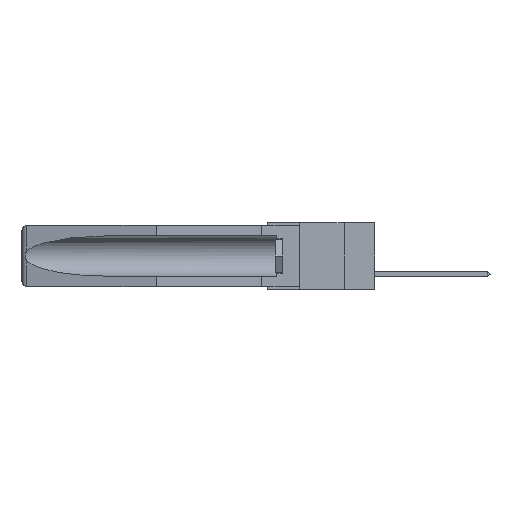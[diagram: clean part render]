
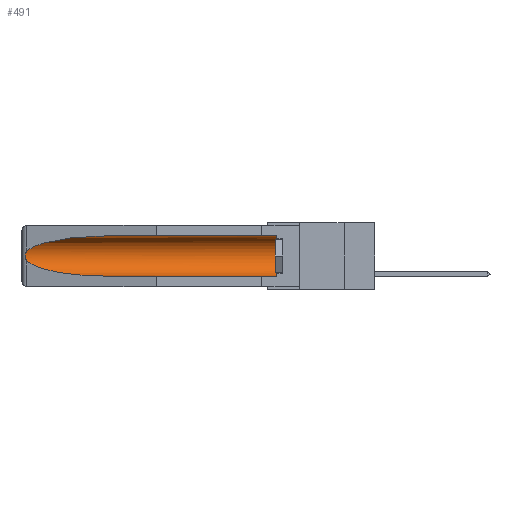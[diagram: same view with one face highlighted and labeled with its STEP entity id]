
A CAD part, left-side view. The second image highlights one B-rep face of the part: STEP entity #491.
In plain terms, the highlighted cylindrical face has radius 2.857 mm (diameter 5.715 mm), a partial arc.
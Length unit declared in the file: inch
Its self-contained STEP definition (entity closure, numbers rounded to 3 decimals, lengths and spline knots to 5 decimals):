
#352 = VERTEX_POINT ( 'NONE', #27739 ) ;
#491 = ADVANCED_FACE ( 'NONE', ( #23785 ), #9913, .F. ) ;
#625 =( BOUNDED_CURVE ( )  B_SPLINE_CURVE ( 3, ( #20214, #18277, #15750, #11184 ),
 .UNSPECIFIED., .F., .F. ) 
 B_SPLINE_CURVE_WITH_KNOTS ( ( 4, 4 ),
 ( 0.1948, 1.5708 ),
 .UNSPECIFIED. ) 
 CURVE ( )  GEOMETRIC_REPRESENTATION_ITEM ( )  RATIONAL_B_SPLINE_CURVE ( ( 1., 0.848, 0.848, 1. ) ) 
 REPRESENTATION_ITEM ( '' )  );
#1029 = DIRECTION ( 'NONE',  ( 0., -1., 0. ) ) ;
#1042 = CARTESIAN_POINT ( 'NONE',  ( 0.26537, 1.52718, -0.14972 ) ) ;
#1168 = CARTESIAN_POINT ( 'NONE',  ( 0.155, 0.126, -0.284 ) ) ;
#1497 = ORIENTED_EDGE ( 'NONE', *, *, #26198, .T. ) ;
#1573 = VECTOR ( 'NONE', #19853, 39.37008 ) ;
#1651 = LINE ( 'NONE', #2618, #8540 ) ;
#1716 = ORIENTED_EDGE ( 'NONE', *, *, #5373, .T. ) ;
#2210 = DIRECTION ( 'NONE',  ( 0., 1., 0. ) ) ;
#2618 = CARTESIAN_POINT ( 'NONE',  ( 0.155, -0.30754, -0.059 ) ) ;
#3207 =( BOUNDED_CURVE ( )  B_SPLINE_CURVE ( 3, ( #17246, #3321, #19295, #7699 ),
 .UNSPECIFIED., .F., .F. ) 
 B_SPLINE_CURVE_WITH_KNOTS ( ( 4, 4 ),
 ( 4.71239, 6.08839 ),
 .UNSPECIFIED. ) 
 CURVE ( )  GEOMETRIC_REPRESENTATION_ITEM ( )  RATIONAL_B_SPLINE_CURVE ( ( 1., 0.848, 0.848, 1. ) ) 
 REPRESENTATION_ITEM ( '' )  );
#3249 = DIRECTION ( 'NONE',  ( 0., 0., 1. ) ) ;
#3321 = CARTESIAN_POINT ( 'NONE',  ( 0.21114, 1.30732, -0.059 ) ) ;
#5340 = CARTESIAN_POINT ( 'NONE',  ( 0.26537, 1.52718, -0.14972 ) ) ;
#5373 = EDGE_CURVE ( 'NONE', #10308, #18978, #3207, .T. ) ;
#5548 = VERTEX_POINT ( 'NONE', #1168 ) ;
#5572 = CARTESIAN_POINT ( 'NONE',  ( 0.26537, 1.52718, -0.19328 ) ) ;
#7217 = EDGE_CURVE ( 'NONE', #5548, #17097, #23941, .T. ) ;
#7699 = CARTESIAN_POINT ( 'NONE',  ( 0.26537, 1.52718, -0.14972 ) ) ;
#8540 = VECTOR ( 'NONE', #25902, 39.37008 ) ;
#9514 = DIRECTION ( 'NONE',  ( 0., 0., 1. ) ) ;
#9913 = CYLINDRICAL_SURFACE ( 'NONE', #21701, 0.1125 ) ;
#10308 = VERTEX_POINT ( 'NONE', #27043 ) ;
#10378 = CARTESIAN_POINT ( 'NONE',  ( 0.2675, 1.53308, -0.16763 ) ) ;
#10491 = CARTESIAN_POINT ( 'NONE',  ( 0.26654, 1.53092, -0.15636 ) ) ;
#11184 = CARTESIAN_POINT ( 'NONE',  ( 0.155, 1.07973, -0.284 ) ) ;
#12759 = CARTESIAN_POINT ( 'NONE',  ( 0.26655, 1.53094, -0.18657 ) ) ;
#12856 = CARTESIAN_POINT ( 'NONE',  ( 0.26537, 1.52718, -0.19328 ) ) ;
#13064 = CARTESIAN_POINT ( 'NONE',  ( 0.2675, 1.53308, -0.17534 ) ) ;
#13317 = B_SPLINE_CURVE_WITH_KNOTS ( 'NONE', 3,
 ( #1042, #22092, #10491, #26961, #10378, #13064, #26656, #12759, #28989, #12856 ),
 .UNSPECIFIED., .F., .F.,
 ( 4, 2, 2, 2, 4 ),
 ( 0., 0.00029, 0.00058, 0.00087, 0.00117 ),
 .UNSPECIFIED. ) ;
#13391 = ORIENTED_EDGE ( 'NONE', *, *, #27439, .T. ) ;
#13919 = CARTESIAN_POINT ( 'NONE',  ( 0.155, -0.30754, -0.1715 ) ) ;
#14907 = CARTESIAN_POINT ( 'NONE',  ( 0.155, -0.30754, -0.284 ) ) ;
#15750 = CARTESIAN_POINT ( 'NONE',  ( 0.21114, 1.30732, -0.284 ) ) ;
#15822 = CARTESIAN_POINT ( 'NONE',  ( 0.155, 0.126, -0.059 ) ) ;
#17097 = VERTEX_POINT ( 'NONE', #15822 ) ;
#17246 = CARTESIAN_POINT ( 'NONE',  ( 0.155, 1.07973, -0.059 ) ) ;
#17316 = VERTEX_POINT ( 'NONE', #5572 ) ;
#18277 = CARTESIAN_POINT ( 'NONE',  ( 0.25451, 1.48313, -0.24835 ) ) ;
#18835 = EDGE_CURVE ( 'NONE', #17316, #352, #625, .T. ) ;
#18978 = VERTEX_POINT ( 'NONE', #5340 ) ;
#19295 = CARTESIAN_POINT ( 'NONE',  ( 0.25451, 1.48313, -0.09465 ) ) ;
#19853 = DIRECTION ( 'NONE',  ( 0., 1., 0. ) ) ;
#20214 = CARTESIAN_POINT ( 'NONE',  ( 0.26537, 1.52718, -0.19328 ) ) ;
#21607 = AXIS2_PLACEMENT_3D ( 'NONE', #26747, #1029, #3249 ) ;
#21701 = AXIS2_PLACEMENT_3D ( 'NONE', #13919, #2210, #9514 ) ;
#22092 = CARTESIAN_POINT ( 'NONE',  ( 0.26597, 1.52961, -0.15275 ) ) ;
#22108 = ORIENTED_EDGE ( 'NONE', *, *, #25700, .F. ) ;
#23785 = FACE_OUTER_BOUND ( 'NONE', #26765, .T. ) ;
#23941 = CIRCLE ( 'NONE', #21607, 0.1125 ) ;
#25700 = EDGE_CURVE ( 'NONE', #5548, #352, #28830, .T. ) ;
#25902 = DIRECTION ( 'NONE',  ( 0., 1., 0. ) ) ;
#25970 = ORIENTED_EDGE ( 'NONE', *, *, #7217, .T. ) ;
#26198 = EDGE_CURVE ( 'NONE', #18978, #17316, #13317, .T. ) ;
#26656 = CARTESIAN_POINT ( 'NONE',  ( 0.2673, 1.53269, -0.17917 ) ) ;
#26747 = CARTESIAN_POINT ( 'NONE',  ( 0.155, 0.126, -0.1715 ) ) ;
#26765 = EDGE_LOOP ( 'NONE', ( #1716, #1497, #28994, #22108, #25970, #13391 ) ) ;
#26961 = CARTESIAN_POINT ( 'NONE',  ( 0.2673, 1.5327, -0.16383 ) ) ;
#27043 = CARTESIAN_POINT ( 'NONE',  ( 0.155, 1.07973, -0.059 ) ) ;
#27439 = EDGE_CURVE ( 'NONE', #17097, #10308, #1651, .T. ) ;
#27739 = CARTESIAN_POINT ( 'NONE',  ( 0.155, 1.07973, -0.284 ) ) ;
#28830 = LINE ( 'NONE', #14907, #1573 ) ;
#28989 = CARTESIAN_POINT ( 'NONE',  ( 0.26597, 1.5296, -0.19026 ) ) ;
#28994 = ORIENTED_EDGE ( 'NONE', *, *, #18835, .T. ) ;
